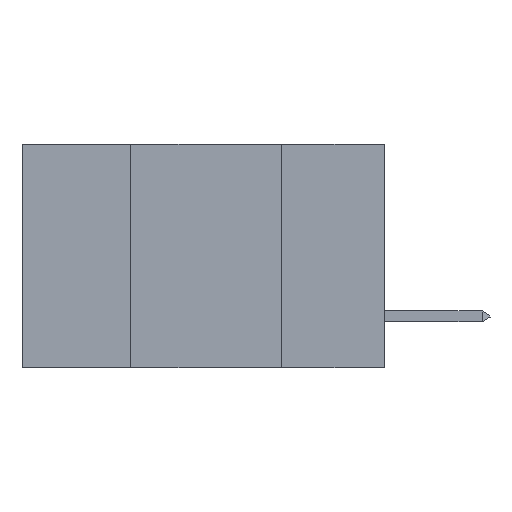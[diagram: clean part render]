
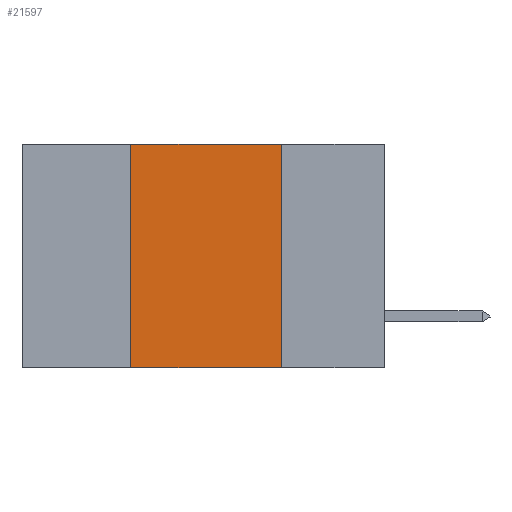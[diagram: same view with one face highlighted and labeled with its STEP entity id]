
A CAD part, left-side view. The second image highlights one B-rep face of the part: STEP entity #21597.
In plain terms, the highlighted planar face has unit normal (-1, 0, 0).
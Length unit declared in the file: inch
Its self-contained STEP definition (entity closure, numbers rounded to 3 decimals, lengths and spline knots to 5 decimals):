
#1357 = ORIENTED_EDGE ( 'NONE', *, *, #20069, .F. ) ;
#1875 = CARTESIAN_POINT ( 'NONE',  ( 0., 0.42, -0.37 ) ) ;
#2103 = AXIS2_PLACEMENT_3D ( 'NONE', #12555, #2602, #18461 ) ;
#2602 = DIRECTION ( 'NONE',  ( 1., 0., 0. ) ) ;
#3237 = ORIENTED_EDGE ( 'NONE', *, *, #15696, .T. ) ;
#3713 = CARTESIAN_POINT ( 'NONE',  ( 0., 0.42, 0. ) ) ;
#3912 = LINE ( 'NONE', #9911, #12292 ) ;
#4234 = DIRECTION ( 'NONE',  ( 0., -1., 0. ) ) ;
#4497 = DIRECTION ( 'NONE',  ( 0., 0., -1. ) ) ;
#5203 = VERTEX_POINT ( 'NONE', #14281 ) ;
#5519 = DIRECTION ( 'NONE',  ( 0., 0., 1. ) ) ;
#7793 = VECTOR ( 'NONE', #5519, 39.37008 ) ;
#8325 = CARTESIAN_POINT ( 'NONE',  ( 0., 0.17, 0. ) ) ;
#9389 = EDGE_LOOP ( 'NONE', ( #18133, #24325, #1357, #3237 ) ) ;
#9911 = CARTESIAN_POINT ( 'NONE',  ( 0., 0.6, -0.37 ) ) ;
#10809 = DIRECTION ( 'NONE',  ( 0., -1., 0. ) ) ;
#12292 = VECTOR ( 'NONE', #4234, 39.37008 ) ;
#12555 = CARTESIAN_POINT ( 'NONE',  ( 0., 0.6, 0. ) ) ;
#13132 = LINE ( 'NONE', #8325, #23324 ) ;
#14281 = CARTESIAN_POINT ( 'NONE',  ( 0., 0.17, 0. ) ) ;
#15696 = EDGE_CURVE ( 'NONE', #16981, #25300, #3912, .T. ) ;
#16521 = CARTESIAN_POINT ( 'NONE',  ( 0., 0.17, -0.37 ) ) ;
#16560 = CARTESIAN_POINT ( 'NONE',  ( 0., 0.6, 0. ) ) ;
#16842 = VECTOR ( 'NONE', #10809, 39.37008 ) ;
#16981 = VERTEX_POINT ( 'NONE', #1875 ) ;
#17684 = EDGE_CURVE ( 'NONE', #19615, #5203, #19916, .T. ) ;
#18081 = EDGE_CURVE ( 'NONE', #5203, #25300, #13132, .T. ) ;
#18133 = ORIENTED_EDGE ( 'NONE', *, *, #18081, .F. ) ;
#18461 = DIRECTION ( 'NONE',  ( 0., 0., -1. ) ) ;
#18550 = PLANE ( 'NONE',  #2103 ) ;
#18578 = FACE_OUTER_BOUND ( 'NONE', #9389, .T. ) ;
#19615 = VERTEX_POINT ( 'NONE', #3713 ) ;
#19916 = LINE ( 'NONE', #16560, #16842 ) ;
#20069 = EDGE_CURVE ( 'NONE', #16981, #19615, #23594, .T. ) ;
#21597 = ADVANCED_FACE ( 'NONE', ( #18578 ), #18550, .F. ) ;
#23324 = VECTOR ( 'NONE', #4497, 39.37008 ) ;
#23440 = CARTESIAN_POINT ( 'NONE',  ( 0., 0.42, 0. ) ) ;
#23594 = LINE ( 'NONE', #23440, #7793 ) ;
#24325 = ORIENTED_EDGE ( 'NONE', *, *, #17684, .F. ) ;
#25300 = VERTEX_POINT ( 'NONE', #16521 ) ;
